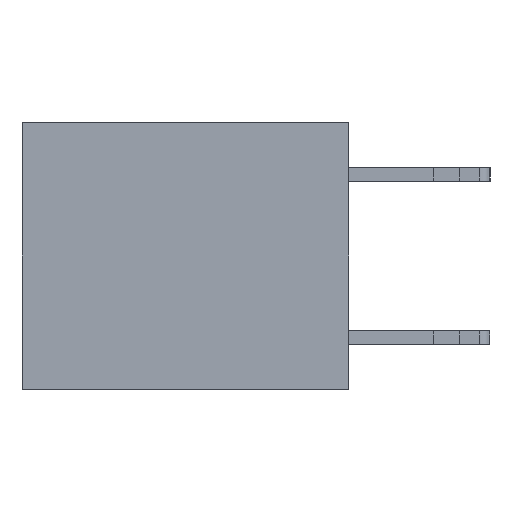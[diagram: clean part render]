
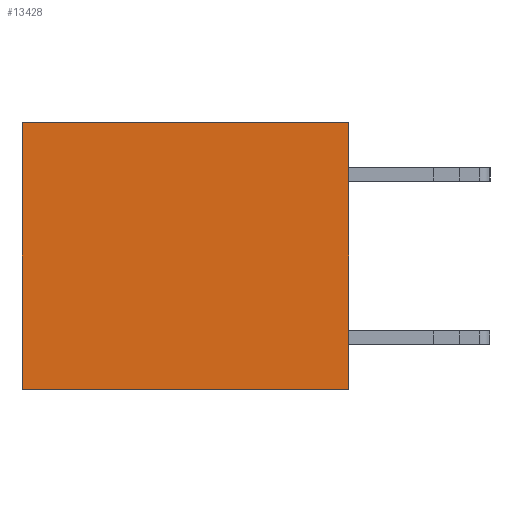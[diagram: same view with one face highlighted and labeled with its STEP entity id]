
A CAD part, left-side view. The second image highlights one B-rep face of the part: STEP entity #13428.
In plain terms, the highlighted planar face has unit normal (-1, 0, 0).
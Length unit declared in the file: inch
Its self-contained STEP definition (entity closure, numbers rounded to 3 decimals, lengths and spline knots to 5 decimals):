
#105 = AXIS2_PLACEMENT_3D ( 'NONE', #9169, #3504, #13729 ) ;
#796 = LINE ( 'NONE', #12468, #4464 ) ;
#835 = VECTOR ( 'NONE', #13643, 39.37008 ) ;
#2270 = ORIENTED_EDGE ( 'NONE', *, *, #10743, .F. ) ;
#2292 = LINE ( 'NONE', #18315, #16949 ) ;
#2499 = DIRECTION ( 'NONE',  ( 0., 0., -1. ) ) ;
#3390 = LINE ( 'NONE', #7895, #835 ) ;
#3504 = DIRECTION ( 'NONE',  ( 1., 0., 0. ) ) ;
#3588 = DIRECTION ( 'NONE',  ( 0., 0., -1. ) ) ;
#3624 = DIRECTION ( 'NONE',  ( 0., 1., 0. ) ) ;
#4193 = CARTESIAN_POINT ( 'NONE',  ( 0.3165, 0.6, -0.49 ) ) ;
#4464 = VECTOR ( 'NONE', #3624, 39.37008 ) ;
#5709 = EDGE_CURVE ( 'NONE', #17677, #13992, #3390, .T. ) ;
#6581 = ORIENTED_EDGE ( 'NONE', *, *, #5709, .T. ) ;
#6599 = EDGE_CURVE ( 'NONE', #12619, #17329, #796, .T. ) ;
#7895 = CARTESIAN_POINT ( 'NONE',  ( 0.3165, 0., 0. ) ) ;
#8340 = EDGE_LOOP ( 'NONE', ( #17534, #8363, #2270, #6581 ) ) ;
#8363 = ORIENTED_EDGE ( 'NONE', *, *, #6599, .F. ) ;
#8368 = CARTESIAN_POINT ( 'NONE',  ( 0.3165, 0.6, -0.49 ) ) ;
#9169 = CARTESIAN_POINT ( 'NONE',  ( 0.3165, 0., -0.49 ) ) ;
#10339 = VECTOR ( 'NONE', #2499, 39.37008 ) ;
#10743 = EDGE_CURVE ( 'NONE', #17677, #12619, #2292, .T. ) ;
#11180 = CARTESIAN_POINT ( 'NONE',  ( 0.3165, 0.6, 0. ) ) ;
#12125 = PLANE ( 'NONE',  #105 ) ;
#12468 = CARTESIAN_POINT ( 'NONE',  ( 0.3165, 0., -0.49 ) ) ;
#12619 = VERTEX_POINT ( 'NONE', #17179 ) ;
#13428 = ADVANCED_FACE ( 'NONE', ( #14100 ), #12125, .F. ) ;
#13643 = DIRECTION ( 'NONE',  ( 0., 1., 0. ) ) ;
#13729 = DIRECTION ( 'NONE',  ( 0., 0., -1. ) ) ;
#13992 = VERTEX_POINT ( 'NONE', #11180 ) ;
#14100 = FACE_OUTER_BOUND ( 'NONE', #8340, .T. ) ;
#14257 = LINE ( 'NONE', #8368, #10339 ) ;
#14983 = EDGE_CURVE ( 'NONE', #13992, #17329, #14257, .T. ) ;
#15199 = CARTESIAN_POINT ( 'NONE',  ( 0.3165, 0., 0. ) ) ;
#16949 = VECTOR ( 'NONE', #3588, 39.37008 ) ;
#17179 = CARTESIAN_POINT ( 'NONE',  ( 0.3165, 0., -0.49 ) ) ;
#17329 = VERTEX_POINT ( 'NONE', #4193 ) ;
#17534 = ORIENTED_EDGE ( 'NONE', *, *, #14983, .T. ) ;
#17677 = VERTEX_POINT ( 'NONE', #15199 ) ;
#18315 = CARTESIAN_POINT ( 'NONE',  ( 0.3165, 0., -0.49 ) ) ;
